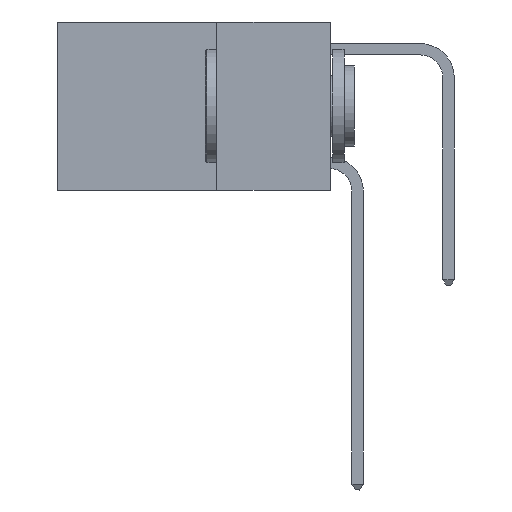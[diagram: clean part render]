
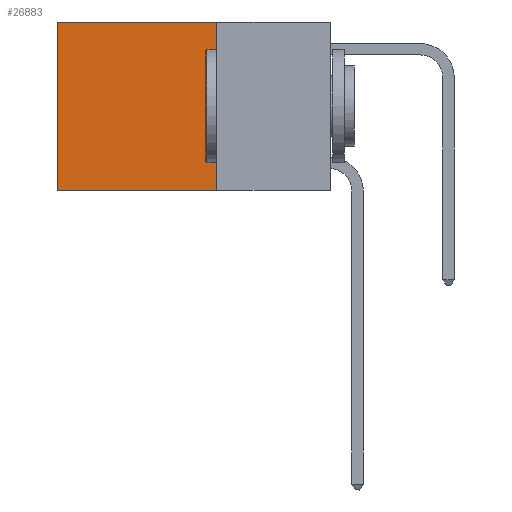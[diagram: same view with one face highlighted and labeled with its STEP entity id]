
A CAD part, left-side view. The second image highlights one B-rep face of the part: STEP entity #26883.
In plain terms, the highlighted planar face has unit normal (-1, 0, 0).
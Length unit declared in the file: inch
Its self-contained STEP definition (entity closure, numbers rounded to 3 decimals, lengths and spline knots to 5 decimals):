
#1641 = DIRECTION ( 'NONE',  ( 0., 1., 0. ) ) ;
#2048 = LINE ( 'NONE', #28353, #18409 ) ;
#2105 = EDGE_CURVE ( 'NONE', #4882, #10763, #7710, .T. ) ;
#3150 = CARTESIAN_POINT ( 'NONE',  ( 0.2625, 0.6, 0. ) ) ;
#3474 = ORIENTED_EDGE ( 'NONE', *, *, #12975, .T. ) ;
#4396 = VERTEX_POINT ( 'NONE', #5176 ) ;
#4505 = DIRECTION ( 'NONE',  ( 0., 0., -1. ) ) ;
#4882 = VERTEX_POINT ( 'NONE', #30424 ) ;
#5176 = CARTESIAN_POINT ( 'NONE',  ( 0.2625, 0.25, -0.37 ) ) ;
#5873 = FACE_OUTER_BOUND ( 'NONE', #32271, .T. ) ;
#7202 = AXIS2_PLACEMENT_3D ( 'NONE', #14679, #19768, #4505 ) ;
#7710 = LINE ( 'NONE', #15991, #32801 ) ;
#10763 = VERTEX_POINT ( 'NONE', #3150 ) ;
#11651 = DIRECTION ( 'NONE',  ( 0., 1., 0. ) ) ;
#11814 = CARTESIAN_POINT ( 'NONE',  ( 0.2625, 0.25, -0.37 ) ) ;
#12067 = ORIENTED_EDGE ( 'NONE', *, *, #2105, .T. ) ;
#12975 = EDGE_CURVE ( 'NONE', #10763, #15218, #25563, .T. ) ;
#13489 = DIRECTION ( 'NONE',  ( 0., 0., -1. ) ) ;
#14115 = EDGE_CURVE ( 'NONE', #4882, #4396, #2048, .T. ) ;
#14679 = CARTESIAN_POINT ( 'NONE',  ( 0.2625, 0.25, 0. ) ) ;
#15218 = VERTEX_POINT ( 'NONE', #32924 ) ;
#15991 = CARTESIAN_POINT ( 'NONE',  ( 0.2625, 0.25, 0. ) ) ;
#16704 = VECTOR ( 'NONE', #1641, 39.37008 ) ;
#18409 = VECTOR ( 'NONE', #20748, 39.37008 ) ;
#19768 = DIRECTION ( 'NONE',  ( 1., 0., 0. ) ) ;
#20748 = DIRECTION ( 'NONE',  ( 0., 0., -1. ) ) ;
#23207 = ORIENTED_EDGE ( 'NONE', *, *, #25977, .F. ) ;
#23440 = LINE ( 'NONE', #11814, #16704 ) ;
#24794 = PLANE ( 'NONE',  #7202 ) ;
#25563 = LINE ( 'NONE', #28518, #31920 ) ;
#25977 = EDGE_CURVE ( 'NONE', #4396, #15218, #23440, .T. ) ;
#26883 = ADVANCED_FACE ( 'NONE', ( #5873 ), #24794, .F. ) ;
#27161 = ORIENTED_EDGE ( 'NONE', *, *, #14115, .F. ) ;
#28353 = CARTESIAN_POINT ( 'NONE',  ( 0.2625, 0.25, 0. ) ) ;
#28518 = CARTESIAN_POINT ( 'NONE',  ( 0.2625, 0.6, 0. ) ) ;
#30424 = CARTESIAN_POINT ( 'NONE',  ( 0.2625, 0.25, 0. ) ) ;
#31920 = VECTOR ( 'NONE', #13489, 39.37008 ) ;
#32271 = EDGE_LOOP ( 'NONE', ( #3474, #23207, #27161, #12067 ) ) ;
#32801 = VECTOR ( 'NONE', #11651, 39.37008 ) ;
#32924 = CARTESIAN_POINT ( 'NONE',  ( 0.2625, 0.6, -0.37 ) ) ;
